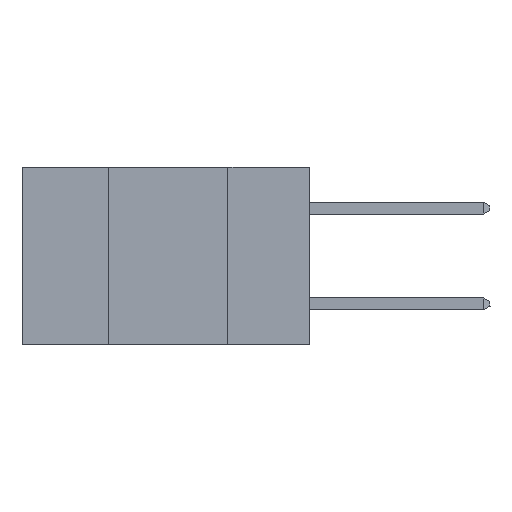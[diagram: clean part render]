
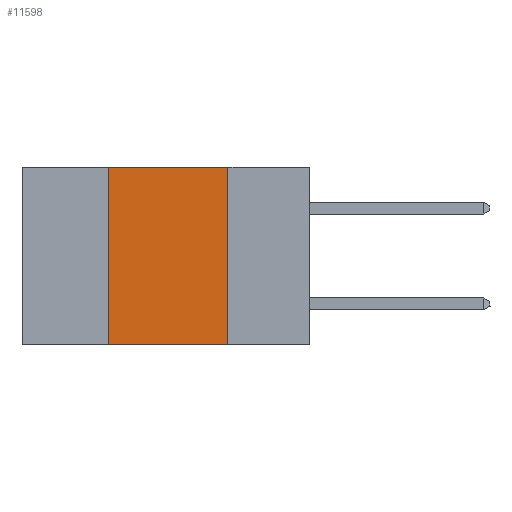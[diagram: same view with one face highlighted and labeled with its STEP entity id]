
A CAD part, left-side view. The second image highlights one B-rep face of the part: STEP entity #11598.
In plain terms, the highlighted planar face has unit normal (-1, 0, 0).
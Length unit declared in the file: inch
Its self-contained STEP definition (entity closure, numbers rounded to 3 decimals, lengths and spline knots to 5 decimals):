
#1080 = ORIENTED_EDGE ( 'NONE', *, *, #16426, .F. ) ;
#1503 = VECTOR ( 'NONE', #23647, 39.37008 ) ;
#1984 = FACE_OUTER_BOUND ( 'NONE', #33637, .T. ) ;
#9724 = ORIENTED_EDGE ( 'NONE', *, *, #36130, .F. ) ;
#10229 = EDGE_CURVE ( 'NONE', #23761, #29065, #29712, .T. ) ;
#11598 = ADVANCED_FACE ( 'NONE', ( #1984 ), #30409, .F. ) ;
#12194 = CARTESIAN_POINT ( 'NONE',  ( 0., 0.6, 0. ) ) ;
#12575 = DIRECTION ( 'NONE',  ( 1., 0., 0. ) ) ;
#14642 = LINE ( 'NONE', #29267, #23664 ) ;
#15662 = CARTESIAN_POINT ( 'NONE',  ( 0., 0.42, -0.37 ) ) ;
#16426 = EDGE_CURVE ( 'NONE', #29011, #23761, #33599, .T. ) ;
#16801 = LINE ( 'NONE', #29546, #1503 ) ;
#17036 = DIRECTION ( 'NONE',  ( 0., 0., 1. ) ) ;
#19237 = VECTOR ( 'NONE', #33346, 39.37008 ) ;
#19507 = CARTESIAN_POINT ( 'NONE',  ( 0., 0.42, 0. ) ) ;
#20016 = ORIENTED_EDGE ( 'NONE', *, *, #21127, .T. ) ;
#21127 = EDGE_CURVE ( 'NONE', #29011, #28850, #14642, .T. ) ;
#21756 = CARTESIAN_POINT ( 'NONE',  ( 0., 0.17, -0.37 ) ) ;
#23644 = AXIS2_PLACEMENT_3D ( 'NONE', #12194, #12575, #33895 ) ;
#23647 = DIRECTION ( 'NONE',  ( 0., 0., -1. ) ) ;
#23664 = VECTOR ( 'NONE', #26183, 39.37008 ) ;
#23761 = VERTEX_POINT ( 'NONE', #19507 ) ;
#25214 = CARTESIAN_POINT ( 'NONE',  ( 0., 0.17, 0. ) ) ;
#26183 = DIRECTION ( 'NONE',  ( 0., -1., 0. ) ) ;
#27351 = VECTOR ( 'NONE', #17036, 39.37008 ) ;
#28850 = VERTEX_POINT ( 'NONE', #21756 ) ;
#29011 = VERTEX_POINT ( 'NONE', #15662 ) ;
#29065 = VERTEX_POINT ( 'NONE', #25214 ) ;
#29267 = CARTESIAN_POINT ( 'NONE',  ( 0., 0.6, -0.37 ) ) ;
#29546 = CARTESIAN_POINT ( 'NONE',  ( 0., 0.17, 0. ) ) ;
#29712 = LINE ( 'NONE', #36522, #19237 ) ;
#30409 = PLANE ( 'NONE',  #23644 ) ;
#33346 = DIRECTION ( 'NONE',  ( 0., -1., 0. ) ) ;
#33599 = LINE ( 'NONE', #35540, #27351 ) ;
#33637 = EDGE_LOOP ( 'NONE', ( #9724, #36539, #1080, #20016 ) ) ;
#33895 = DIRECTION ( 'NONE',  ( 0., 0., -1. ) ) ;
#35540 = CARTESIAN_POINT ( 'NONE',  ( 0., 0.42, 0. ) ) ;
#36130 = EDGE_CURVE ( 'NONE', #29065, #28850, #16801, .T. ) ;
#36522 = CARTESIAN_POINT ( 'NONE',  ( 0., 0.6, 0. ) ) ;
#36539 = ORIENTED_EDGE ( 'NONE', *, *, #10229, .F. ) ;
